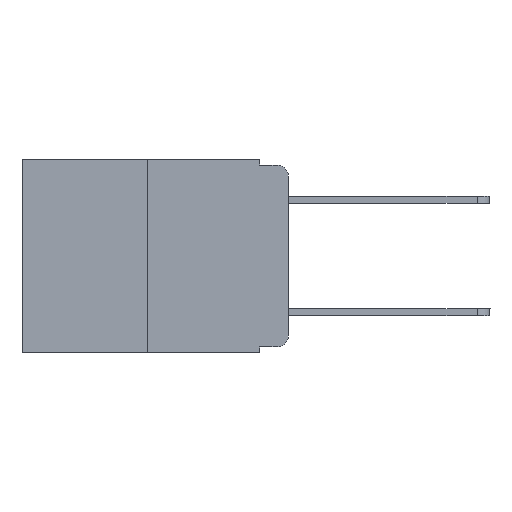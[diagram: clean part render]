
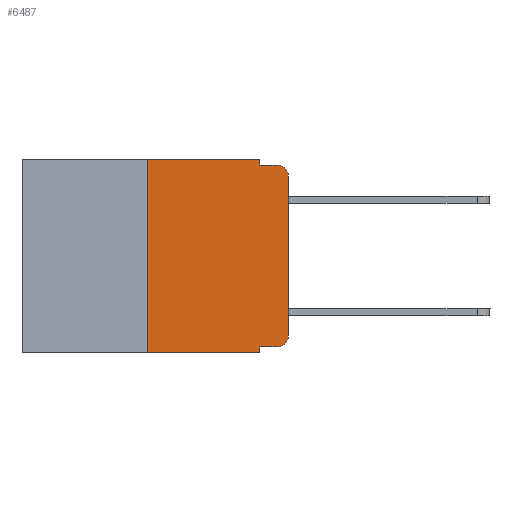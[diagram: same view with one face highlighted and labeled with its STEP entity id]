
A CAD part, left-side view. The second image highlights one B-rep face of the part: STEP entity #6487.
In plain terms, the highlighted planar face has unit normal (-1, 0, 0).
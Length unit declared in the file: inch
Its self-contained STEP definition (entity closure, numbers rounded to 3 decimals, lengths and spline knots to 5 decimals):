
#388 = CARTESIAN_POINT ( 'NONE',  ( 0., 0.02, -0.333 ) ) ;
#703 = DIRECTION ( 'NONE',  ( 0., 0., -1. ) ) ;
#1208 = CARTESIAN_POINT ( 'NONE',  ( 0., 0.051, -0.01 ) ) ;
#1558 = VECTOR ( 'NONE', #8870, 39.37008 ) ;
#1571 = CARTESIAN_POINT ( 'NONE',  ( 0., 0., -0.313 ) ) ;
#1618 = EDGE_CURVE ( 'NONE', #4253, #5036, #3709, .T. ) ;
#1684 = VECTOR ( 'NONE', #703, 39.37008 ) ;
#1807 = DIRECTION ( 'NONE',  ( 0., -1., 0. ) ) ;
#1823 = VERTEX_POINT ( 'NONE', #4538 ) ;
#1950 = ORIENTED_EDGE ( 'NONE', *, *, #2209, .T. ) ;
#1984 = ORIENTED_EDGE ( 'NONE', *, *, #9202, .T. ) ;
#2209 = EDGE_CURVE ( 'NONE', #7850, #8565, #9937, .T. ) ;
#2278 = LINE ( 'NONE', #2331, #2799 ) ;
#2331 = CARTESIAN_POINT ( 'NONE',  ( 0., 0.051, 0. ) ) ;
#2427 = DIRECTION ( 'NONE',  ( 0., 0., 1. ) ) ;
#2546 = VERTEX_POINT ( 'NONE', #5200 ) ;
#2799 = VECTOR ( 'NONE', #8147, 39.37008 ) ;
#2854 = CARTESIAN_POINT ( 'NONE',  ( 0., 0.051, 0. ) ) ;
#2880 = ORIENTED_EDGE ( 'NONE', *, *, #4855, .F. ) ;
#3069 = LINE ( 'NONE', #6003, #7134 ) ;
#3338 = VERTEX_POINT ( 'NONE', #6847 ) ;
#3653 = CARTESIAN_POINT ( 'NONE',  ( 0., 0.473, 0. ) ) ;
#3668 = EDGE_CURVE ( 'NONE', #5036, #5138, #9449, .T. ) ;
#3683 = ORIENTED_EDGE ( 'NONE', *, *, #1618, .F. ) ;
#3709 = LINE ( 'NONE', #6606, #1558 ) ;
#3962 = DIRECTION ( 'NONE',  ( -1., 0., 0. ) ) ;
#4023 = DIRECTION ( 'NONE',  ( 0., 0., -1. ) ) ;
#4097 = AXIS2_PLACEMENT_3D ( 'NONE', #7958, #3962, #4023 ) ;
#4119 = CARTESIAN_POINT ( 'NONE',  ( 0., 0.25, -0.343 ) ) ;
#4253 = VERTEX_POINT ( 'NONE', #4119 ) ;
#4299 = LINE ( 'NONE', #8473, #4416 ) ;
#4306 = CARTESIAN_POINT ( 'NONE',  ( 0., 0.25, 0. ) ) ;
#4416 = VECTOR ( 'NONE', #7679, 39.37008 ) ;
#4428 = DIRECTION ( 'NONE',  ( 0., 0., -1. ) ) ;
#4447 = LINE ( 'NONE', #7120, #9675 ) ;
#4538 = CARTESIAN_POINT ( 'NONE',  ( 0., 0.051, -0.333 ) ) ;
#4573 = LINE ( 'NONE', #1208, #7875 ) ;
#4581 = EDGE_CURVE ( 'NONE', #1823, #7850, #3069, .T. ) ;
#4689 = EDGE_LOOP ( 'NONE', ( #1984, #9193, #8602, #2880, #8241, #3683, #5786, #5640, #10138, #1950 ) ) ;
#4853 = EDGE_CURVE ( 'NONE', #7589, #3338, #9684, .T. ) ;
#4855 = EDGE_CURVE ( 'NONE', #5138, #2546, #7398, .T. ) ;
#5036 = VERTEX_POINT ( 'NONE', #4306 ) ;
#5138 = VERTEX_POINT ( 'NONE', #2854 ) ;
#5200 = CARTESIAN_POINT ( 'NONE',  ( 0., 0.051, -0.01 ) ) ;
#5599 = AXIS2_PLACEMENT_3D ( 'NONE', #3653, #9371, #4428 ) ;
#5640 = ORIENTED_EDGE ( 'NONE', *, *, #5655, .F. ) ;
#5655 = EDGE_CURVE ( 'NONE', #1823, #8032, #2278, .T. ) ;
#5786 = ORIENTED_EDGE ( 'NONE', *, *, #7203, .T. ) ;
#5830 = DIRECTION ( 'NONE',  ( 0., 0., -1. ) ) ;
#5997 = DIRECTION ( 'NONE',  ( 0., -1., 0. ) ) ;
#6003 = CARTESIAN_POINT ( 'NONE',  ( 0., 0.051, -0.333 ) ) ;
#6328 = CARTESIAN_POINT ( 'NONE',  ( 0., 0.051, 0. ) ) ;
#6487 = ADVANCED_FACE ( 'NONE', ( #6595 ), #9409, .F. ) ;
#6595 = FACE_OUTER_BOUND ( 'NONE', #4689, .T. ) ;
#6606 = CARTESIAN_POINT ( 'NONE',  ( 0., 0.25, 0. ) ) ;
#6679 = CARTESIAN_POINT ( 'NONE',  ( 0., 0.02, -0.313 ) ) ;
#6847 = CARTESIAN_POINT ( 'NONE',  ( 0., 0.02, -0.01 ) ) ;
#6864 = AXIS2_PLACEMENT_3D ( 'NONE', #6679, #9131, #5830 ) ;
#7120 = CARTESIAN_POINT ( 'NONE',  ( 0., 0., 0. ) ) ;
#7134 = VECTOR ( 'NONE', #7611, 39.37008 ) ;
#7203 = EDGE_CURVE ( 'NONE', #4253, #8032, #4299, .T. ) ;
#7398 = LINE ( 'NONE', #6328, #1684 ) ;
#7589 = VERTEX_POINT ( 'NONE', #9802 ) ;
#7611 = DIRECTION ( 'NONE',  ( 0., -1., 0. ) ) ;
#7679 = DIRECTION ( 'NONE',  ( 0., -1., 0. ) ) ;
#7850 = VERTEX_POINT ( 'NONE', #388 ) ;
#7875 = VECTOR ( 'NONE', #5997, 39.37008 ) ;
#7958 = CARTESIAN_POINT ( 'NONE',  ( 0., 0.02, -0.03 ) ) ;
#8032 = VERTEX_POINT ( 'NONE', #9458 ) ;
#8147 = DIRECTION ( 'NONE',  ( 0., 0., -1. ) ) ;
#8241 = ORIENTED_EDGE ( 'NONE', *, *, #3668, .F. ) ;
#8473 = CARTESIAN_POINT ( 'NONE',  ( 0., 0.473, -0.343 ) ) ;
#8565 = VERTEX_POINT ( 'NONE', #1571 ) ;
#8602 = ORIENTED_EDGE ( 'NONE', *, *, #8977, .F. ) ;
#8870 = DIRECTION ( 'NONE',  ( 0., 0., 1. ) ) ;
#8977 = EDGE_CURVE ( 'NONE', #2546, #3338, #4573, .T. ) ;
#9105 = CARTESIAN_POINT ( 'NONE',  ( 0., 0.473, 0. ) ) ;
#9131 = DIRECTION ( 'NONE',  ( -1., 0., 0. ) ) ;
#9192 = VECTOR ( 'NONE', #1807, 39.37008 ) ;
#9193 = ORIENTED_EDGE ( 'NONE', *, *, #4853, .T. ) ;
#9202 = EDGE_CURVE ( 'NONE', #8565, #7589, #4447, .T. ) ;
#9371 = DIRECTION ( 'NONE',  ( 1., 0., 0. ) ) ;
#9409 = PLANE ( 'NONE',  #5599 ) ;
#9449 = LINE ( 'NONE', #9105, #9192 ) ;
#9458 = CARTESIAN_POINT ( 'NONE',  ( 0., 0.051, -0.343 ) ) ;
#9675 = VECTOR ( 'NONE', #2427, 39.37008 ) ;
#9684 = CIRCLE ( 'NONE', #4097, 0.02 ) ;
#9802 = CARTESIAN_POINT ( 'NONE',  ( 0., 0., -0.03 ) ) ;
#9937 = CIRCLE ( 'NONE', #6864, 0.02 ) ;
#10138 = ORIENTED_EDGE ( 'NONE', *, *, #4581, .T. ) ;
